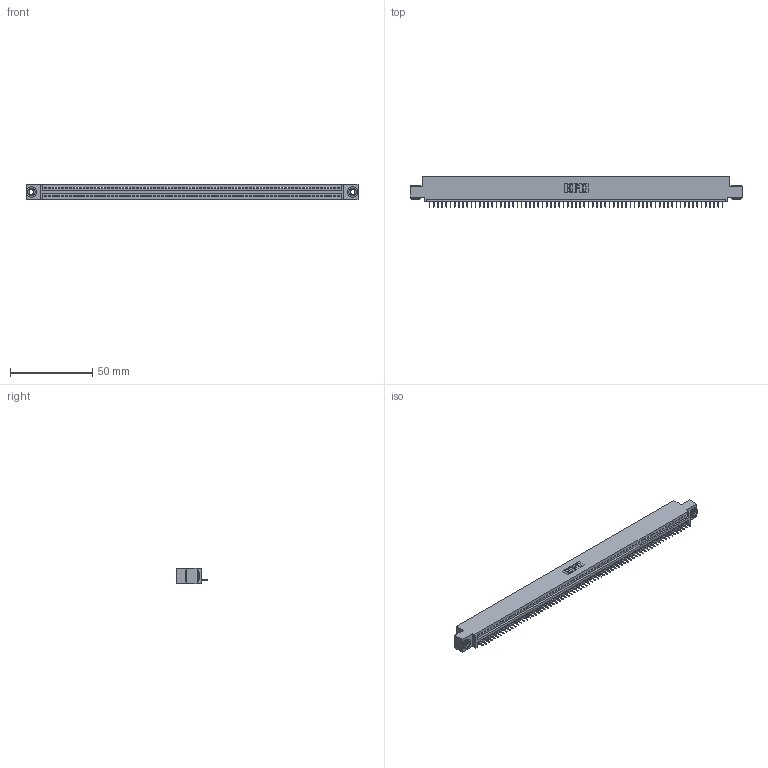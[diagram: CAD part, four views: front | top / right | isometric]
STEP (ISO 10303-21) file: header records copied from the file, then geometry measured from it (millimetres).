
FILE_DESCRIPTION (( 'STEP AP203' ), '1' );
FILE_NAME ('345-071-525-403.STEP', '2020-09-21T08:36:50', ( '' ), ( '' ), 'SwSTEP 2.0', 'SolidWorks 2020', '' );
FILE_SCHEMA (( 'CONFIG_CONTROL_DESIGN' ));
Length unit declared in the file: inch
Products named in the file (4): 345-250-002_345-250-002-102; 345-292-001_345-293-125; 345 Part_0.110 Offset - 0.156 Dia-TH; 345-071-525-403
Assembly tree (74 placements, depth 2):
  345-071-525-403
    345 Part_0.110 Offset - 0.156 Dia-TH
    345-292-001_345-293-125  x71
    345-250-002_345-250-002-102  x2
Bounding box: 201.55 x 18.72 x 9.4 mm (x, y, z)
Volume: 19037 mm3; surface area: 25022.3 mm2
Topology: 74 solids, 74 shells, 4570 faces, 13209 edges, 8518 vertices
Faces by surface type: plane 3360, cylinder 1202, cone 8
Entity records: 50388 total; most frequent: CARTESIAN_POINT 8704, ORIENTED_EDGE 8702, DIRECTION 7591, EDGE_CURVE 4351, LINE 3915, VECTOR 3915, VERTEX_POINT 2894, AXIS2_PLACEMENT_3D 1838
